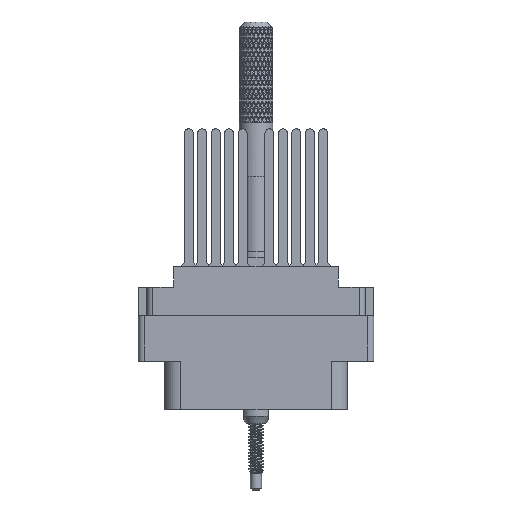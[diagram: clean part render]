
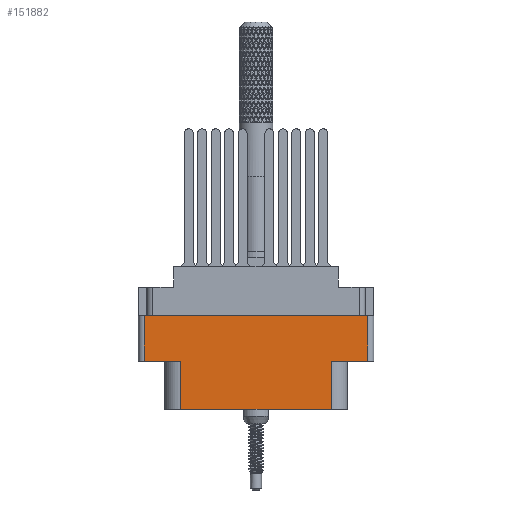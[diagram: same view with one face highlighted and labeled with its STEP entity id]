
A CAD part, front view. The second image highlights one B-rep face of the part: STEP entity #151882.
In plain terms, the highlighted planar face has unit normal (0, -1, 0).
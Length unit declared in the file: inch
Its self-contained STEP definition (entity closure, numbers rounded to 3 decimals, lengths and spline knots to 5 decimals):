
#9038 = ORIENTED_EDGE ( 'NONE', *, *, #169441, .T. ) ;
#9460 = VERTEX_POINT ( 'NONE', #86636 ) ;
#9833 = VERTEX_POINT ( 'NONE', #78745 ) ;
#17303 = LINE ( 'NONE', #29117, #30917 ) ;
#17361 = VERTEX_POINT ( 'NONE', #114123 ) ;
#18629 = EDGE_CURVE ( 'NONE', #17361, #162185, #130192, .T. ) ;
#21905 = DIRECTION ( 'NONE',  ( 0., 0., -1. ) ) ;
#24545 = VERTEX_POINT ( 'NONE', #49497 ) ;
#28281 = VECTOR ( 'NONE', #50956, 39.37008 ) ;
#29117 = CARTESIAN_POINT ( 'NONE',  ( 0., -0.343, -0.274 ) ) ;
#30917 = VECTOR ( 'NONE', #158994, 39.37008 ) ;
#33695 = LINE ( 'NONE', #135543, #40406 ) ;
#40406 = VECTOR ( 'NONE', #77941, 39.37008 ) ;
#42507 = AXIS2_PLACEMENT_3D ( 'NONE', #63649, #78867, #21905 ) ;
#43975 = EDGE_LOOP ( 'NONE', ( #123111, #147990, #9038, #156698, #97933, #128115, #112702, #82922 ) ) ;
#44849 = CARTESIAN_POINT ( 'NONE',  ( -0.42052, -0.343, -0.798 ) ) ;
#49497 = CARTESIAN_POINT ( 'NONE',  ( -0.42052, -0.343, -0.529 ) ) ;
#50956 = DIRECTION ( 'NONE',  ( 0., 0., -1. ) ) ;
#51593 = FACE_OUTER_BOUND ( 'NONE', #43975, .T. ) ;
#55224 = EDGE_CURVE ( 'NONE', #17361, #126212, #100585, .T. ) ;
#55506 = DIRECTION ( 'NONE',  ( 0., 0., 1. ) ) ;
#58027 = DIRECTION ( 'NONE',  ( 1., 0., 0. ) ) ;
#59996 = VECTOR ( 'NONE', #55506, 39.37008 ) ;
#60990 = DIRECTION ( 'NONE',  ( 0., 0., 1. ) ) ;
#63649 = CARTESIAN_POINT ( 'NONE',  ( -0.656, -0.343, -0.798 ) ) ;
#66088 = VECTOR ( 'NONE', #58027, 39.37008 ) ;
#75178 = LINE ( 'NONE', #146634, #66088 ) ;
#77941 = DIRECTION ( 'NONE',  ( 1., 0., 0. ) ) ;
#78745 = CARTESIAN_POINT ( 'NONE',  ( 0.42052, -0.343, -0.798 ) ) ;
#78867 = DIRECTION ( 'NONE',  ( 0., -1., 0. ) ) ;
#80522 = CARTESIAN_POINT ( 'NONE',  ( -0.42052, -0.343, -0.798 ) ) ;
#82922 = ORIENTED_EDGE ( 'NONE', *, *, #55224, .T. ) ;
#83077 = LINE ( 'NONE', #80522, #85280 ) ;
#83841 = CARTESIAN_POINT ( 'NONE',  ( 0.42052, -0.343, -0.529 ) ) ;
#84847 = EDGE_CURVE ( 'NONE', #9460, #153856, #150546, .T. ) ;
#85280 = VECTOR ( 'NONE', #124199, 39.37008 ) ;
#86636 = CARTESIAN_POINT ( 'NONE',  ( -0.624, -0.343, -0.274 ) ) ;
#91390 = CARTESIAN_POINT ( 'NONE',  ( 0.624, -0.343, -0.798 ) ) ;
#97933 = ORIENTED_EDGE ( 'NONE', *, *, #165844, .T. ) ;
#98485 = VERTEX_POINT ( 'NONE', #44849 ) ;
#100585 = LINE ( 'NONE', #91390, #147932 ) ;
#112702 = ORIENTED_EDGE ( 'NONE', *, *, #18629, .F. ) ;
#114123 = CARTESIAN_POINT ( 'NONE',  ( 0.624, -0.343, -0.529 ) ) ;
#116282 = CARTESIAN_POINT ( 'NONE',  ( 0.42052, -0.343, -0.529 ) ) ;
#116934 = CARTESIAN_POINT ( 'NONE',  ( 0., -0.343, -0.529 ) ) ;
#120671 = PLANE ( 'NONE',  #42507 ) ;
#123111 = ORIENTED_EDGE ( 'NONE', *, *, #126991, .F. ) ;
#124199 = DIRECTION ( 'NONE',  ( 0., 0., -1. ) ) ;
#126212 = VERTEX_POINT ( 'NONE', #142389 ) ;
#126799 = EDGE_CURVE ( 'NONE', #24545, #98485, #83077, .T. ) ;
#126991 = EDGE_CURVE ( 'NONE', #9460, #126212, #17303, .T. ) ;
#128115 = ORIENTED_EDGE ( 'NONE', *, *, #139204, .T. ) ;
#130192 = LINE ( 'NONE', #116934, #155116 ) ;
#135543 = CARTESIAN_POINT ( 'NONE',  ( 0., -0.343, -0.529 ) ) ;
#139204 = EDGE_CURVE ( 'NONE', #9833, #162185, #152957, .T. ) ;
#142389 = CARTESIAN_POINT ( 'NONE',  ( 0.624, -0.343, -0.274 ) ) ;
#146634 = CARTESIAN_POINT ( 'NONE',  ( -0.656, -0.343, -0.798 ) ) ;
#147932 = VECTOR ( 'NONE', #60990, 39.37008 ) ;
#147990 = ORIENTED_EDGE ( 'NONE', *, *, #84847, .T. ) ;
#150546 = LINE ( 'NONE', #151681, #28281 ) ;
#151681 = CARTESIAN_POINT ( 'NONE',  ( -0.624, -0.343, -0.798 ) ) ;
#151686 = CARTESIAN_POINT ( 'NONE',  ( -0.624, -0.343, -0.529 ) ) ;
#151882 = ADVANCED_FACE ( 'NONE', ( #51593 ), #120671, .T. ) ;
#152957 = LINE ( 'NONE', #116282, #59996 ) ;
#153856 = VERTEX_POINT ( 'NONE', #151686 ) ;
#155116 = VECTOR ( 'NONE', #176387, 39.37008 ) ;
#156698 = ORIENTED_EDGE ( 'NONE', *, *, #126799, .T. ) ;
#158994 = DIRECTION ( 'NONE',  ( 1., 0., 0. ) ) ;
#162185 = VERTEX_POINT ( 'NONE', #83841 ) ;
#165844 = EDGE_CURVE ( 'NONE', #98485, #9833, #75178, .T. ) ;
#169441 = EDGE_CURVE ( 'NONE', #153856, #24545, #33695, .T. ) ;
#176387 = DIRECTION ( 'NONE',  ( -1., 0., 0. ) ) ;
